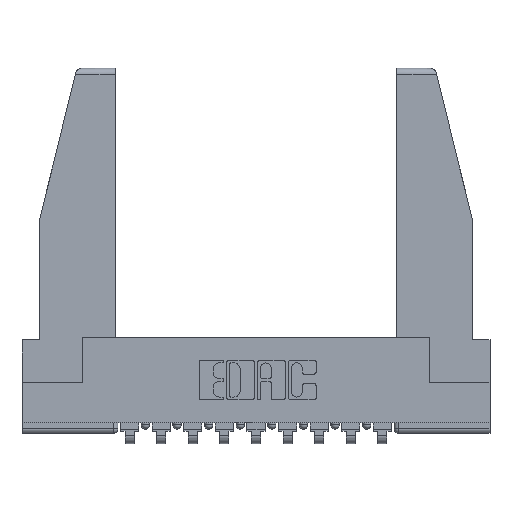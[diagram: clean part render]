
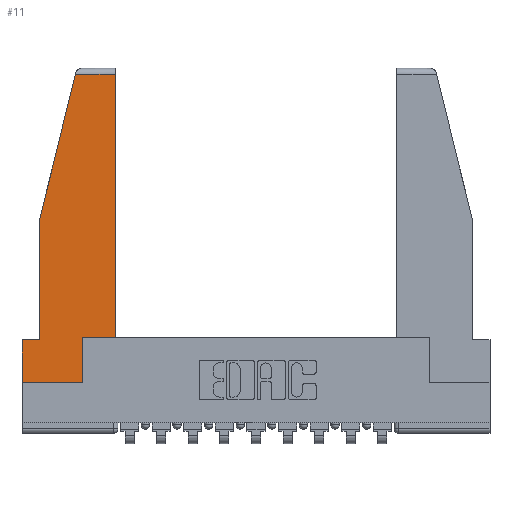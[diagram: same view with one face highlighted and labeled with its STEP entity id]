
A CAD part, top view. The second image highlights one B-rep face of the part: STEP entity #11.
In plain terms, the highlighted planar face has unit normal (0, 0, 1).
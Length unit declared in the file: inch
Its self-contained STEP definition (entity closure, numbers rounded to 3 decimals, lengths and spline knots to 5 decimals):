
#11 = ADVANCED_FACE ( 'NONE', ( #5443 ), #9164, .T. ) ;
#460 = DIRECTION ( 'NONE',  ( 0., -1., 0. ) ) ;
#579 = VECTOR ( 'NONE', #6884, 39.37008 ) ;
#773 = CARTESIAN_POINT ( 'NONE',  ( 0., 0., 0. ) ) ;
#1018 = EDGE_CURVE ( 'NONE', #6837, #7764, #13646, .T. ) ;
#1150 = LINE ( 'NONE', #3496, #14994 ) ;
#1286 = LINE ( 'NONE', #11910, #1966 ) ;
#1482 = ORIENTED_EDGE ( 'NONE', *, *, #3570, .T. ) ;
#1483 = DIRECTION ( 'NONE',  ( -0.239, -0.971, 0. ) ) ;
#1794 = EDGE_CURVE ( 'NONE', #8577, #9208, #1286, .T. ) ;
#1966 = VECTOR ( 'NONE', #13050, 39.37008 ) ;
#1981 = ORIENTED_EDGE ( 'NONE', *, *, #10735, .T. ) ;
#1998 = VERTEX_POINT ( 'NONE', #11421 ) ;
#2136 = CARTESIAN_POINT ( 'NONE',  ( 0.086, 0.21, 0. ) ) ;
#2148 = LINE ( 'NONE', #8080, #579 ) ;
#2163 = ORIENTED_EDGE ( 'NONE', *, *, #1794, .T. ) ;
#2392 = CARTESIAN_POINT ( 'NONE',  ( 0., 0., 0. ) ) ;
#2584 = CARTESIAN_POINT ( 'NONE',  ( 0.297, 0.223, 0. ) ) ;
#2691 = CARTESIAN_POINT ( 'NONE',  ( 0.271, 1.55, 0. ) ) ;
#2734 = VECTOR ( 'NONE', #5764, 39.37008 ) ;
#2901 = VERTEX_POINT ( 'NONE', #8001 ) ;
#3152 = CARTESIAN_POINT ( 'NONE',  ( 0.461, 0.223, 0. ) ) ;
#3218 = DIRECTION ( 'NONE',  ( 1., 0., 0. ) ) ;
#3496 = CARTESIAN_POINT ( 'NONE',  ( 0., 1.52, 0. ) ) ;
#3549 = VECTOR ( 'NONE', #1483, 39.37008 ) ;
#3570 = EDGE_CURVE ( 'NONE', #14221, #5867, #10860, .T. ) ;
#3609 = LINE ( 'NONE', #7965, #2734 ) ;
#3763 = EDGE_CURVE ( 'NONE', #5867, #8577, #3609, .T. ) ;
#3890 = LINE ( 'NONE', #2584, #7193 ) ;
#3947 = EDGE_LOOP ( 'NONE', ( #14639, #11608, #1482, #14102, #2163, #14824, #1981, #13701, #6127 ) ) ;
#4194 = CARTESIAN_POINT ( 'NONE',  ( 0., 0.21, 0. ) ) ;
#4261 = EDGE_CURVE ( 'NONE', #2901, #1998, #2148, .T. ) ;
#4291 = EDGE_CURVE ( 'NONE', #7764, #14221, #1150, .T. ) ;
#4783 = VERTEX_POINT ( 'NONE', #2392 ) ;
#4972 = DIRECTION ( 'NONE',  ( 1., 0., 0. ) ) ;
#5277 = LINE ( 'NONE', #4194, #14986 ) ;
#5343 = CARTESIAN_POINT ( 'NONE',  ( 0.2636, 1.52, 0. ) ) ;
#5443 = FACE_OUTER_BOUND ( 'NONE', #3947, .T. ) ;
#5764 = DIRECTION ( 'NONE',  ( 0., -1., 0. ) ) ;
#5867 = VERTEX_POINT ( 'NONE', #6682 ) ;
#6127 = ORIENTED_EDGE ( 'NONE', *, *, #7019, .T. ) ;
#6200 = AXIS2_PLACEMENT_3D ( 'NONE', #773, #8941, #3218 ) ;
#6652 = EDGE_CURVE ( 'NONE', #9208, #4783, #5277, .T. ) ;
#6682 = CARTESIAN_POINT ( 'NONE',  ( 0.086, 0.8, 0. ) ) ;
#6837 = VERTEX_POINT ( 'NONE', #9155 ) ;
#6884 = DIRECTION ( 'NONE',  ( 0., 1., 0. ) ) ;
#7019 = EDGE_CURVE ( 'NONE', #1998, #6837, #3890, .T. ) ;
#7193 = VECTOR ( 'NONE', #10529, 39.37008 ) ;
#7764 = VERTEX_POINT ( 'NONE', #10926 ) ;
#7965 = CARTESIAN_POINT ( 'NONE',  ( 0.086, 0.8, 0. ) ) ;
#8001 = CARTESIAN_POINT ( 'NONE',  ( 0.297, 0., 0. ) ) ;
#8080 = CARTESIAN_POINT ( 'NONE',  ( 0.297, 0., 0. ) ) ;
#8577 = VERTEX_POINT ( 'NONE', #2136 ) ;
#8941 = DIRECTION ( 'NONE',  ( 0., 0., 1. ) ) ;
#9155 = CARTESIAN_POINT ( 'NONE',  ( 0.461, 0.223, 0. ) ) ;
#9164 = PLANE ( 'NONE',  #6200 ) ;
#9208 = VERTEX_POINT ( 'NONE', #13025 ) ;
#9609 = CARTESIAN_POINT ( 'NONE',  ( 0., 0., 0. ) ) ;
#9648 = VECTOR ( 'NONE', #4972, 39.37008 ) ;
#10528 = DIRECTION ( 'NONE',  ( -1., 0., 0. ) ) ;
#10529 = DIRECTION ( 'NONE',  ( 1., 0., 0. ) ) ;
#10735 = EDGE_CURVE ( 'NONE', #4783, #2901, #14388, .T. ) ;
#10860 = LINE ( 'NONE', #2691, #3549 ) ;
#10926 = CARTESIAN_POINT ( 'NONE',  ( 0.461, 1.52, 0. ) ) ;
#11421 = CARTESIAN_POINT ( 'NONE',  ( 0.297, 0.223, 0. ) ) ;
#11608 = ORIENTED_EDGE ( 'NONE', *, *, #4291, .T. ) ;
#11910 = CARTESIAN_POINT ( 'NONE',  ( 0., 0.21, 0. ) ) ;
#13025 = CARTESIAN_POINT ( 'NONE',  ( 0., 0.21, 0. ) ) ;
#13050 = DIRECTION ( 'NONE',  ( -1., 0., 0. ) ) ;
#13646 = LINE ( 'NONE', #3152, #14695 ) ;
#13701 = ORIENTED_EDGE ( 'NONE', *, *, #4261, .T. ) ;
#14102 = ORIENTED_EDGE ( 'NONE', *, *, #3763, .T. ) ;
#14221 = VERTEX_POINT ( 'NONE', #5343 ) ;
#14388 = LINE ( 'NONE', #9609, #9648 ) ;
#14639 = ORIENTED_EDGE ( 'NONE', *, *, #1018, .T. ) ;
#14695 = VECTOR ( 'NONE', #14775, 39.37008 ) ;
#14775 = DIRECTION ( 'NONE',  ( 0., 1., 0. ) ) ;
#14824 = ORIENTED_EDGE ( 'NONE', *, *, #6652, .T. ) ;
#14986 = VECTOR ( 'NONE', #460, 39.37008 ) ;
#14994 = VECTOR ( 'NONE', #10528, 39.37008 ) ;
